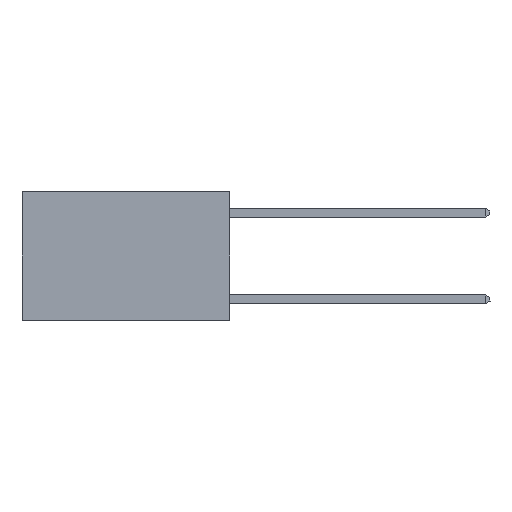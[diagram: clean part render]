
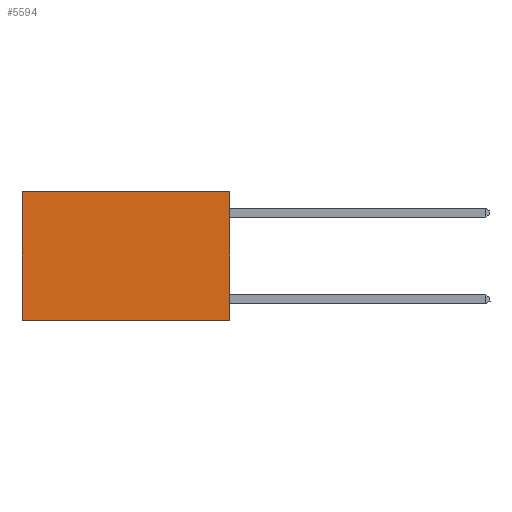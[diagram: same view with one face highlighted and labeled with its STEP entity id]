
A CAD part, left-side view. The second image highlights one B-rep face of the part: STEP entity #5594.
In plain terms, the highlighted planar face has unit normal (-1, 0, 0).
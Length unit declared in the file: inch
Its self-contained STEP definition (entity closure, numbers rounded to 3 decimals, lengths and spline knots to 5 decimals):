
#327 = CARTESIAN_POINT ( 'NONE',  ( 0.2625, 0.6, 0. ) ) ;
#1067 = DIRECTION ( 'NONE',  ( 0., 0., -1. ) ) ;
#2700 = VERTEX_POINT ( 'NONE', #16008 ) ;
#2748 = ORIENTED_EDGE ( 'NONE', *, *, #4751, .F. ) ;
#2918 = EDGE_CURVE ( 'NONE', #2700, #16432, #10367, .T. ) ;
#3203 = VECTOR ( 'NONE', #3514, 39.37008 ) ;
#3462 = CARTESIAN_POINT ( 'NONE',  ( 0.2625, 0.6, -0.37 ) ) ;
#3514 = DIRECTION ( 'NONE',  ( 0., 0., -1. ) ) ;
#4061 = VECTOR ( 'NONE', #13754, 39.37008 ) ;
#4162 = VERTEX_POINT ( 'NONE', #327 ) ;
#4297 = ORIENTED_EDGE ( 'NONE', *, *, #5488, .T. ) ;
#4745 = LINE ( 'NONE', #4773, #13951 ) ;
#4751 = EDGE_CURVE ( 'NONE', #11719, #2700, #12014, .T. ) ;
#4773 = CARTESIAN_POINT ( 'NONE',  ( 0.2625, 0., 0. ) ) ;
#5488 = EDGE_CURVE ( 'NONE', #4162, #16432, #14887, .T. ) ;
#5594 = ADVANCED_FACE ( 'NONE', ( #9650 ), #13641, .F. ) ;
#7324 = CARTESIAN_POINT ( 'NONE',  ( 0.2625, 0., -0.37 ) ) ;
#7849 = CARTESIAN_POINT ( 'NONE',  ( 0.2625, 0., 0. ) ) ;
#7917 = EDGE_LOOP ( 'NONE', ( #4297, #15152, #2748, #10148 ) ) ;
#8676 = DIRECTION ( 'NONE',  ( 0., 1., 0. ) ) ;
#9650 = FACE_OUTER_BOUND ( 'NONE', #7917, .T. ) ;
#9716 = CARTESIAN_POINT ( 'NONE',  ( 0.2625, 0., 0. ) ) ;
#10148 = ORIENTED_EDGE ( 'NONE', *, *, #13258, .T. ) ;
#10367 = LINE ( 'NONE', #7324, #12461 ) ;
#11719 = VERTEX_POINT ( 'NONE', #15259 ) ;
#11862 = DIRECTION ( 'NONE',  ( 1., 0., 0. ) ) ;
#12014 = LINE ( 'NONE', #9716, #4061 ) ;
#12461 = VECTOR ( 'NONE', #8676, 39.37008 ) ;
#13258 = EDGE_CURVE ( 'NONE', #11719, #4162, #4745, .T. ) ;
#13641 = PLANE ( 'NONE',  #16549 ) ;
#13754 = DIRECTION ( 'NONE',  ( 0., 0., -1. ) ) ;
#13951 = VECTOR ( 'NONE', #15790, 39.37008 ) ;
#14887 = LINE ( 'NONE', #16764, #3203 ) ;
#15152 = ORIENTED_EDGE ( 'NONE', *, *, #2918, .F. ) ;
#15259 = CARTESIAN_POINT ( 'NONE',  ( 0.2625, 0., 0. ) ) ;
#15790 = DIRECTION ( 'NONE',  ( 0., 1., 0. ) ) ;
#16008 = CARTESIAN_POINT ( 'NONE',  ( 0.2625, 0., -0.37 ) ) ;
#16432 = VERTEX_POINT ( 'NONE', #3462 ) ;
#16549 = AXIS2_PLACEMENT_3D ( 'NONE', #7849, #11862, #1067 ) ;
#16764 = CARTESIAN_POINT ( 'NONE',  ( 0.2625, 0.6, 0. ) ) ;
